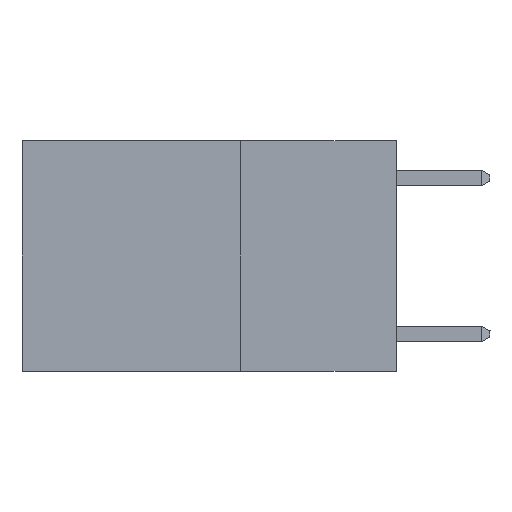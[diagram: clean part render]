
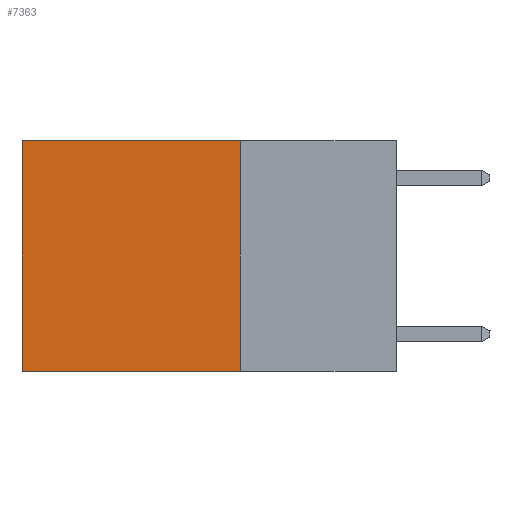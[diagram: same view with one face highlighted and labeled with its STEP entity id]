
A CAD part, left-side view. The second image highlights one B-rep face of the part: STEP entity #7363.
In plain terms, the highlighted planar face has unit normal (-1, 0, 0).
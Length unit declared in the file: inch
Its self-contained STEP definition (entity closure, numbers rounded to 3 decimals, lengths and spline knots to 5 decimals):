
#296 = CARTESIAN_POINT ( 'NONE',  ( 0.2625, 0.25, -0.37 ) ) ;
#394 = EDGE_LOOP ( 'NONE', ( #2153, #6028, #9697, #9772 ) ) ;
#579 = LINE ( 'NONE', #9977, #5820 ) ;
#809 = AXIS2_PLACEMENT_3D ( 'NONE', #3574, #2062, #8571 ) ;
#847 = FACE_OUTER_BOUND ( 'NONE', #394, .T. ) ;
#1862 = CARTESIAN_POINT ( 'NONE',  ( 0.2625, 0.25, 0. ) ) ;
#2062 = DIRECTION ( 'NONE',  ( 1., 0., 0. ) ) ;
#2153 = ORIENTED_EDGE ( 'NONE', *, *, #3885, .T. ) ;
#2181 = LINE ( 'NONE', #7197, #3703 ) ;
#2193 = VECTOR ( 'NONE', #3050, 39.37008 ) ;
#3019 = CARTESIAN_POINT ( 'NONE',  ( 0.2625, 0.25, 0. ) ) ;
#3050 = DIRECTION ( 'NONE',  ( 0., 0., -1. ) ) ;
#3116 = DIRECTION ( 'NONE',  ( 0., 1., 0. ) ) ;
#3573 = VERTEX_POINT ( 'NONE', #1862 ) ;
#3574 = CARTESIAN_POINT ( 'NONE',  ( 0.2625, 0.25, 0. ) ) ;
#3579 = LINE ( 'NONE', #3019, #2193 ) ;
#3703 = VECTOR ( 'NONE', #3116, 39.37008 ) ;
#3885 = EDGE_CURVE ( 'NONE', #4788, #5947, #4254, .T. ) ;
#4068 = CARTESIAN_POINT ( 'NONE',  ( 0.2625, 0.6, 0. ) ) ;
#4254 = LINE ( 'NONE', #7996, #10431 ) ;
#4453 = PLANE ( 'NONE',  #809 ) ;
#4788 = VERTEX_POINT ( 'NONE', #4068 ) ;
#4871 = EDGE_CURVE ( 'NONE', #3573, #4788, #2181, .T. ) ;
#5120 = VERTEX_POINT ( 'NONE', #296 ) ;
#5820 = VECTOR ( 'NONE', #6017, 39.37008 ) ;
#5947 = VERTEX_POINT ( 'NONE', #8682 ) ;
#6017 = DIRECTION ( 'NONE',  ( 0., 1., 0. ) ) ;
#6028 = ORIENTED_EDGE ( 'NONE', *, *, #7272, .F. ) ;
#6392 = DIRECTION ( 'NONE',  ( 0., 0., -1. ) ) ;
#7197 = CARTESIAN_POINT ( 'NONE',  ( 0.2625, 0.25, 0. ) ) ;
#7272 = EDGE_CURVE ( 'NONE', #5120, #5947, #579, .T. ) ;
#7363 = ADVANCED_FACE ( 'NONE', ( #847 ), #4453, .F. ) ;
#7996 = CARTESIAN_POINT ( 'NONE',  ( 0.2625, 0.6, 0. ) ) ;
#8571 = DIRECTION ( 'NONE',  ( 0., 0., -1. ) ) ;
#8682 = CARTESIAN_POINT ( 'NONE',  ( 0.2625, 0.6, -0.37 ) ) ;
#9646 = EDGE_CURVE ( 'NONE', #3573, #5120, #3579, .T. ) ;
#9697 = ORIENTED_EDGE ( 'NONE', *, *, #9646, .F. ) ;
#9772 = ORIENTED_EDGE ( 'NONE', *, *, #4871, .T. ) ;
#9977 = CARTESIAN_POINT ( 'NONE',  ( 0.2625, 0.25, -0.37 ) ) ;
#10431 = VECTOR ( 'NONE', #6392, 39.37008 ) ;
